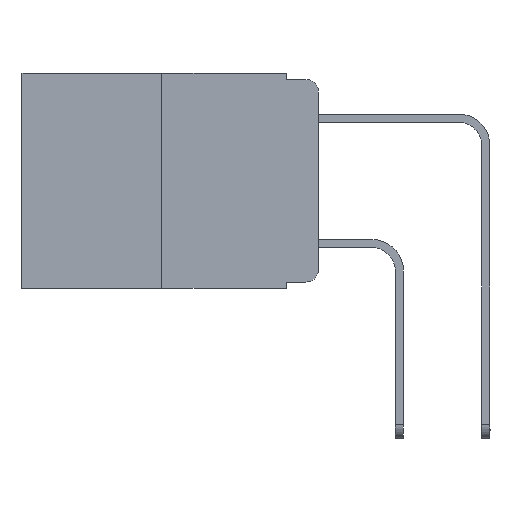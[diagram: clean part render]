
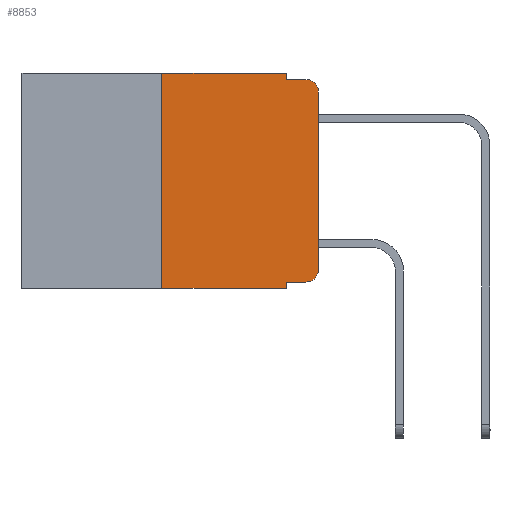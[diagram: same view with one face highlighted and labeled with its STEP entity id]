
A CAD part, left-side view. The second image highlights one B-rep face of the part: STEP entity #8853.
In plain terms, the highlighted planar face has unit normal (-1, 0, 0).
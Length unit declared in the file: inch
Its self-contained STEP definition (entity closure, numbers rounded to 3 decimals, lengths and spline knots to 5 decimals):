
#366 = LINE ( 'NONE', #18666, #20723 ) ;
#542 = AXIS2_PLACEMENT_3D ( 'NONE', #8707, #20282, #8526 ) ;
#1523 = LINE ( 'NONE', #2217, #7947 ) ;
#1682 = EDGE_CURVE ( 'NONE', #6259, #1882, #9568, .T. ) ;
#1882 = VERTEX_POINT ( 'NONE', #23336 ) ;
#2206 = VERTEX_POINT ( 'NONE', #14319 ) ;
#2217 = CARTESIAN_POINT ( 'NONE',  ( 0., 0.051, 0. ) ) ;
#3231 = CARTESIAN_POINT ( 'NONE',  ( 0., 0.051, -0.01 ) ) ;
#4216 = VECTOR ( 'NONE', #9208, 39.37008 ) ;
#4298 = ORIENTED_EDGE ( 'NONE', *, *, #8979, .F. ) ;
#4347 = CIRCLE ( 'NONE', #542, 0.02 ) ;
#4563 = EDGE_CURVE ( 'NONE', #12595, #7180, #22066, .T. ) ;
#4930 = VERTEX_POINT ( 'NONE', #22451 ) ;
#4962 = DIRECTION ( 'NONE',  ( 0., 0., -1. ) ) ;
#4970 = DIRECTION ( 'NONE',  ( 0., -1., 0. ) ) ;
#5398 = EDGE_CURVE ( 'NONE', #4930, #1882, #4347, .T. ) ;
#6127 = CARTESIAN_POINT ( 'NONE',  ( 0., 0.25, 0. ) ) ;
#6259 = VERTEX_POINT ( 'NONE', #16237 ) ;
#6541 = VECTOR ( 'NONE', #10450, 39.37008 ) ;
#6822 = ORIENTED_EDGE ( 'NONE', *, *, #16860, .T. ) ;
#7134 = EDGE_CURVE ( 'NONE', #17771, #6259, #1523, .T. ) ;
#7159 = LINE ( 'NONE', #10370, #20750 ) ;
#7180 = VERTEX_POINT ( 'NONE', #20390 ) ;
#7322 = CARTESIAN_POINT ( 'NONE',  ( 0., 0.02, -0.333 ) ) ;
#7947 = VECTOR ( 'NONE', #12443, 39.37008 ) ;
#8168 = LINE ( 'NONE', #8577, #12191 ) ;
#8314 = DIRECTION ( 'NONE',  ( 0., 0., 1. ) ) ;
#8526 = DIRECTION ( 'NONE',  ( 0., 0., -1. ) ) ;
#8577 = CARTESIAN_POINT ( 'NONE',  ( 0., 0., 0. ) ) ;
#8707 = CARTESIAN_POINT ( 'NONE',  ( 0., 0.02, -0.03 ) ) ;
#8853 = ADVANCED_FACE ( 'NONE', ( #20881 ), #19718, .F. ) ;
#8979 = EDGE_CURVE ( 'NONE', #19713, #19053, #10332, .T. ) ;
#9208 = DIRECTION ( 'NONE',  ( 0., 0., 1. ) ) ;
#9423 = EDGE_CURVE ( 'NONE', #7180, #4930, #8168, .T. ) ;
#9469 = DIRECTION ( 'NONE',  ( 0., -1., 0. ) ) ;
#9568 = LINE ( 'NONE', #3231, #10817 ) ;
#10332 = LINE ( 'NONE', #15375, #4216 ) ;
#10370 = CARTESIAN_POINT ( 'NONE',  ( 0., 0.051, -0.333 ) ) ;
#10416 = ORIENTED_EDGE ( 'NONE', *, *, #19652, .T. ) ;
#10450 = DIRECTION ( 'NONE',  ( 0., -1., 0. ) ) ;
#10817 = VECTOR ( 'NONE', #9469, 39.37008 ) ;
#11102 = VECTOR ( 'NONE', #4962, 39.37008 ) ;
#11228 = ORIENTED_EDGE ( 'NONE', *, *, #25235, .F. ) ;
#11725 = LINE ( 'NONE', #14821, #11102 ) ;
#12191 = VECTOR ( 'NONE', #8314, 39.37008 ) ;
#12443 = DIRECTION ( 'NONE',  ( 0., 0., -1. ) ) ;
#12595 = VERTEX_POINT ( 'NONE', #7322 ) ;
#12772 = ORIENTED_EDGE ( 'NONE', *, *, #7134, .F. ) ;
#13500 = AXIS2_PLACEMENT_3D ( 'NONE', #25161, #15688, #19372 ) ;
#13651 = ORIENTED_EDGE ( 'NONE', *, *, #4563, .T. ) ;
#14226 = ORIENTED_EDGE ( 'NONE', *, *, #20654, .F. ) ;
#14304 = ORIENTED_EDGE ( 'NONE', *, *, #1682, .F. ) ;
#14319 = CARTESIAN_POINT ( 'NONE',  ( 0., 0.051, -0.333 ) ) ;
#14821 = CARTESIAN_POINT ( 'NONE',  ( 0., 0.051, 0. ) ) ;
#15027 = EDGE_LOOP ( 'NONE', ( #21082, #23794, #14304, #12772, #11228, #4298, #6822, #14226, #10416, #13651 ) ) ;
#15375 = CARTESIAN_POINT ( 'NONE',  ( 0., 0.25, 0. ) ) ;
#15688 = DIRECTION ( 'NONE',  ( 1., 0., 0. ) ) ;
#16186 = CARTESIAN_POINT ( 'NONE',  ( 0., 0.473, 0. ) ) ;
#16237 = CARTESIAN_POINT ( 'NONE',  ( 0., 0.051, -0.01 ) ) ;
#16378 = CARTESIAN_POINT ( 'NONE',  ( 0., 0.02, -0.313 ) ) ;
#16860 = EDGE_CURVE ( 'NONE', #19713, #18706, #366, .T. ) ;
#17514 = CARTESIAN_POINT ( 'NONE',  ( 0., 0.051, 0. ) ) ;
#17771 = VERTEX_POINT ( 'NONE', #17514 ) ;
#18583 = LINE ( 'NONE', #16186, #6541 ) ;
#18666 = CARTESIAN_POINT ( 'NONE',  ( 0., 0.473, -0.343 ) ) ;
#18706 = VERTEX_POINT ( 'NONE', #24393 ) ;
#19053 = VERTEX_POINT ( 'NONE', #6127 ) ;
#19372 = DIRECTION ( 'NONE',  ( 0., 0., -1. ) ) ;
#19652 = EDGE_CURVE ( 'NONE', #2206, #12595, #7159, .T. ) ;
#19713 = VERTEX_POINT ( 'NONE', #24136 ) ;
#19718 = PLANE ( 'NONE',  #13500 ) ;
#20233 = DIRECTION ( 'NONE',  ( 0., -1., 0. ) ) ;
#20282 = DIRECTION ( 'NONE',  ( -1., 0., 0. ) ) ;
#20390 = CARTESIAN_POINT ( 'NONE',  ( 0., 0., -0.313 ) ) ;
#20521 = DIRECTION ( 'NONE',  ( -1., 0., 0. ) ) ;
#20654 = EDGE_CURVE ( 'NONE', #2206, #18706, #11725, .T. ) ;
#20723 = VECTOR ( 'NONE', #4970, 39.37008 ) ;
#20750 = VECTOR ( 'NONE', #20233, 39.37008 ) ;
#20881 = FACE_OUTER_BOUND ( 'NONE', #15027, .T. ) ;
#21082 = ORIENTED_EDGE ( 'NONE', *, *, #9423, .T. ) ;
#22066 = CIRCLE ( 'NONE', #25376, 0.02 ) ;
#22451 = CARTESIAN_POINT ( 'NONE',  ( 0., 0., -0.03 ) ) ;
#22462 = DIRECTION ( 'NONE',  ( 0., 0., -1. ) ) ;
#23336 = CARTESIAN_POINT ( 'NONE',  ( 0., 0.02, -0.01 ) ) ;
#23794 = ORIENTED_EDGE ( 'NONE', *, *, #5398, .T. ) ;
#24136 = CARTESIAN_POINT ( 'NONE',  ( 0., 0.25, -0.343 ) ) ;
#24393 = CARTESIAN_POINT ( 'NONE',  ( 0., 0.051, -0.343 ) ) ;
#25161 = CARTESIAN_POINT ( 'NONE',  ( 0., 0.473, 0. ) ) ;
#25235 = EDGE_CURVE ( 'NONE', #19053, #17771, #18583, .T. ) ;
#25376 = AXIS2_PLACEMENT_3D ( 'NONE', #16378, #20521, #22462 ) ;
